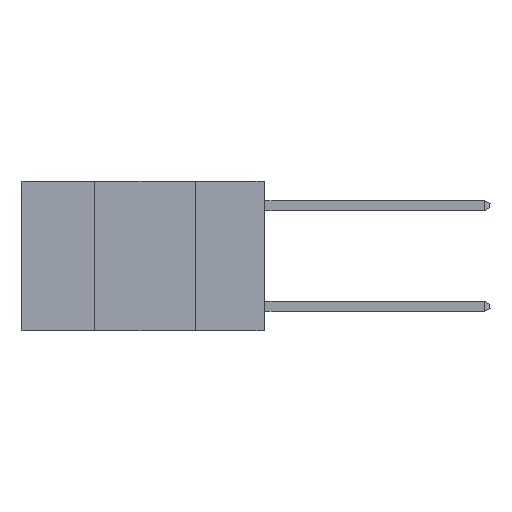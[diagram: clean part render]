
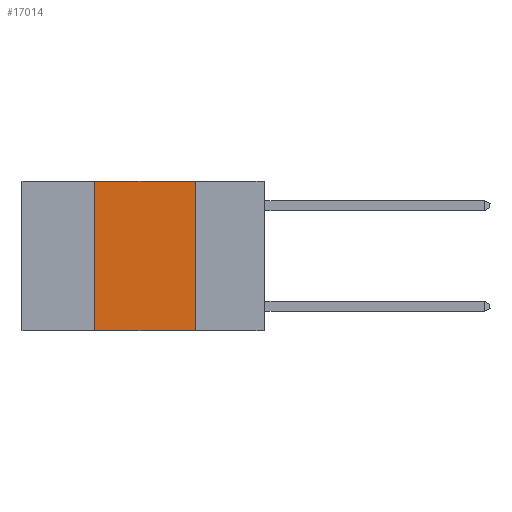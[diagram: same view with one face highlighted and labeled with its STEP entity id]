
A CAD part, left-side view. The second image highlights one B-rep face of the part: STEP entity #17014.
In plain terms, the highlighted planar face has unit normal (-1, 0, 0).
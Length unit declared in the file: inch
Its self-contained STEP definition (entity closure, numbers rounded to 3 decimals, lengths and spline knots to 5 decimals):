
#748 = DIRECTION ( 'NONE',  ( 0., 0., -1. ) ) ;
#1047 = VECTOR ( 'NONE', #6603, 39.37008 ) ;
#2806 = ORIENTED_EDGE ( 'NONE', *, *, #8301, .F. ) ;
#3197 = ORIENTED_EDGE ( 'NONE', *, *, #22604, .F. ) ;
#3331 = DIRECTION ( 'NONE',  ( 0., 0., -1. ) ) ;
#3725 = CARTESIAN_POINT ( 'NONE',  ( 0., 0.6, -0.37 ) ) ;
#5191 = DIRECTION ( 'NONE',  ( 1., 0., 0. ) ) ;
#5628 = CARTESIAN_POINT ( 'NONE',  ( 0., 0.6, 0. ) ) ;
#6603 = DIRECTION ( 'NONE',  ( 0., 0., 1. ) ) ;
#7161 = FACE_OUTER_BOUND ( 'NONE', #16401, .T. ) ;
#8301 = EDGE_CURVE ( 'NONE', #12497, #18611, #16017, .T. ) ;
#8405 = VERTEX_POINT ( 'NONE', #16514 ) ;
#9050 = DIRECTION ( 'NONE',  ( 0., -1., 0. ) ) ;
#9167 = ORIENTED_EDGE ( 'NONE', *, *, #17832, .F. ) ;
#10313 = CARTESIAN_POINT ( 'NONE',  ( 0., 0.17, 0. ) ) ;
#11028 = CARTESIAN_POINT ( 'NONE',  ( 0., 0.17, -0.37 ) ) ;
#11209 = LINE ( 'NONE', #5628, #13831 ) ;
#12083 = EDGE_CURVE ( 'NONE', #12497, #19634, #22329, .T. ) ;
#12099 = AXIS2_PLACEMENT_3D ( 'NONE', #18068, #5191, #3331 ) ;
#12361 = CARTESIAN_POINT ( 'NONE',  ( 0., 0.42, -0.37 ) ) ;
#12497 = VERTEX_POINT ( 'NONE', #12361 ) ;
#12768 = PLANE ( 'NONE',  #12099 ) ;
#13452 = DIRECTION ( 'NONE',  ( 0., -1., 0. ) ) ;
#13831 = VECTOR ( 'NONE', #13452, 39.37008 ) ;
#15633 = LINE ( 'NONE', #10313, #18059 ) ;
#16017 = LINE ( 'NONE', #23582, #1047 ) ;
#16401 = EDGE_LOOP ( 'NONE', ( #9167, #3197, #2806, #18812 ) ) ;
#16514 = CARTESIAN_POINT ( 'NONE',  ( 0., 0.17, 0. ) ) ;
#17014 = ADVANCED_FACE ( 'NONE', ( #7161 ), #12768, .F. ) ;
#17832 = EDGE_CURVE ( 'NONE', #8405, #19634, #15633, .T. ) ;
#18059 = VECTOR ( 'NONE', #748, 39.37008 ) ;
#18068 = CARTESIAN_POINT ( 'NONE',  ( 0., 0.6, 0. ) ) ;
#18611 = VERTEX_POINT ( 'NONE', #18672 ) ;
#18672 = CARTESIAN_POINT ( 'NONE',  ( 0., 0.42, 0. ) ) ;
#18812 = ORIENTED_EDGE ( 'NONE', *, *, #12083, .T. ) ;
#19094 = VECTOR ( 'NONE', #9050, 39.37008 ) ;
#19634 = VERTEX_POINT ( 'NONE', #11028 ) ;
#22329 = LINE ( 'NONE', #3725, #19094 ) ;
#22604 = EDGE_CURVE ( 'NONE', #18611, #8405, #11209, .T. ) ;
#23582 = CARTESIAN_POINT ( 'NONE',  ( 0., 0.42, 0. ) ) ;
